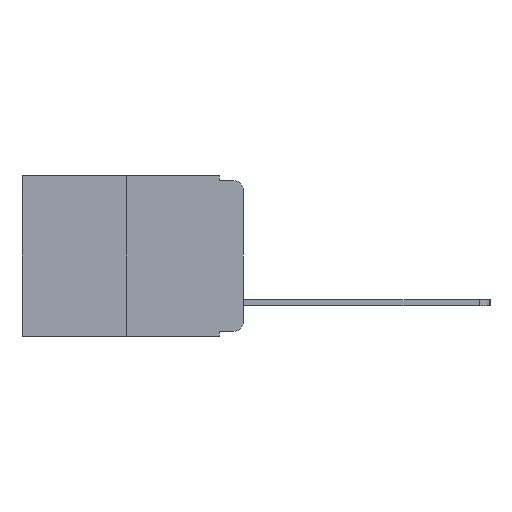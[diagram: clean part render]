
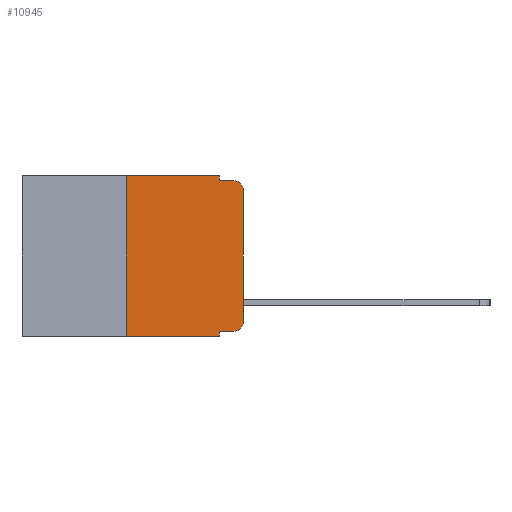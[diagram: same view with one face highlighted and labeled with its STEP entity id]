
A CAD part, left-side view. The second image highlights one B-rep face of the part: STEP entity #10945.
In plain terms, the highlighted planar face has unit normal (-1, 0, 0).
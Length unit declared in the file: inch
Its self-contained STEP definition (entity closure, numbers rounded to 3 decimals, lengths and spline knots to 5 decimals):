
#144 = EDGE_CURVE ( 'NONE', #13487, #6773, #2012, .T. ) ;
#500 = VERTEX_POINT ( 'NONE', #2441 ) ;
#527 = DIRECTION ( 'NONE',  ( 0., -1., 0. ) ) ;
#773 = AXIS2_PLACEMENT_3D ( 'NONE', #11230, #8162, #3846 ) ;
#955 = AXIS2_PLACEMENT_3D ( 'NONE', #4087, #8547, #12707 ) ;
#1427 = CARTESIAN_POINT ( 'NONE',  ( 0., 0.02, -0.01 ) ) ;
#2012 = LINE ( 'NONE', #13451, #7382 ) ;
#2046 = VERTEX_POINT ( 'NONE', #8762 ) ;
#2049 = DIRECTION ( 'NONE',  ( 0., -1., 0. ) ) ;
#2094 = LINE ( 'NONE', #11624, #9943 ) ;
#2283 = ORIENTED_EDGE ( 'NONE', *, *, #3135, .F. ) ;
#2360 = EDGE_LOOP ( 'NONE', ( #12227, #9770, #12539, #10143, #7335, #4859, #7635, #2283, #10321, #7983 ) ) ;
#2441 = CARTESIAN_POINT ( 'NONE',  ( 0., 0.25, -0.343 ) ) ;
#2463 = FACE_OUTER_BOUND ( 'NONE', #2360, .T. ) ;
#3135 = EDGE_CURVE ( 'NONE', #11764, #10428, #8601, .T. ) ;
#3271 = DIRECTION ( 'NONE',  ( 0., 0., 1. ) ) ;
#3550 = VECTOR ( 'NONE', #3271, 39.37008 ) ;
#3846 = DIRECTION ( 'NONE',  ( 0., 0., -1. ) ) ;
#3886 = EDGE_CURVE ( 'NONE', #10408, #6773, #5937, .T. ) ;
#4087 = CARTESIAN_POINT ( 'NONE',  ( 0., 0.473, 0. ) ) ;
#4218 = CARTESIAN_POINT ( 'NONE',  ( 0., 0.25, 0. ) ) ;
#4588 = CARTESIAN_POINT ( 'NONE',  ( 0., 0.02, -0.03 ) ) ;
#4742 = LINE ( 'NONE', #11142, #7216 ) ;
#4859 = ORIENTED_EDGE ( 'NONE', *, *, #9819, .F. ) ;
#4990 = DIRECTION ( 'NONE',  ( 0., 0., -1. ) ) ;
#5002 = DIRECTION ( 'NONE',  ( -1., 0., 0. ) ) ;
#5090 = DIRECTION ( 'NONE',  ( 0., -1., 0. ) ) ;
#5436 = DIRECTION ( 'NONE',  ( 0., 0., -1. ) ) ;
#5575 = VECTOR ( 'NONE', #12709, 39.37008 ) ;
#5848 = EDGE_CURVE ( 'NONE', #2046, #13487, #11241, .T. ) ;
#5937 = CIRCLE ( 'NONE', #10540, 0.02 ) ;
#6435 = EDGE_CURVE ( 'NONE', #500, #10428, #10713, .T. ) ;
#6773 = VERTEX_POINT ( 'NONE', #1427 ) ;
#7216 = VECTOR ( 'NONE', #11431, 39.37008 ) ;
#7335 = ORIENTED_EDGE ( 'NONE', *, *, #12509, .F. ) ;
#7382 = VECTOR ( 'NONE', #5090, 39.37008 ) ;
#7523 = PLANE ( 'NONE',  #955 ) ;
#7635 = ORIENTED_EDGE ( 'NONE', *, *, #6435, .T. ) ;
#7705 = CARTESIAN_POINT ( 'NONE',  ( 0., 0.051, -0.01 ) ) ;
#7826 = EDGE_CURVE ( 'NONE', #8843, #10408, #4742, .T. ) ;
#7895 = VECTOR ( 'NONE', #13499, 39.37008 ) ;
#7983 = ORIENTED_EDGE ( 'NONE', *, *, #10238, .T. ) ;
#7985 = VECTOR ( 'NONE', #5436, 39.37008 ) ;
#8162 = DIRECTION ( 'NONE',  ( -1., 0., 0. ) ) ;
#8256 = CARTESIAN_POINT ( 'NONE',  ( 0., 0.051, 0. ) ) ;
#8547 = DIRECTION ( 'NONE',  ( 1., 0., 0. ) ) ;
#8601 = LINE ( 'NONE', #12526, #7985 ) ;
#8762 = CARTESIAN_POINT ( 'NONE',  ( 0., 0.051, 0. ) ) ;
#8843 = VERTEX_POINT ( 'NONE', #9157 ) ;
#8940 = CIRCLE ( 'NONE', #773, 0.02 ) ;
#9144 = CARTESIAN_POINT ( 'NONE',  ( 0., 0.473, 0. ) ) ;
#9157 = CARTESIAN_POINT ( 'NONE',  ( 0., 0., -0.313 ) ) ;
#9770 = ORIENTED_EDGE ( 'NONE', *, *, #3886, .T. ) ;
#9819 = EDGE_CURVE ( 'NONE', #500, #9896, #11951, .T. ) ;
#9896 = VERTEX_POINT ( 'NONE', #4218 ) ;
#9943 = VECTOR ( 'NONE', #2049, 39.37008 ) ;
#9968 = VERTEX_POINT ( 'NONE', #10446 ) ;
#10143 = ORIENTED_EDGE ( 'NONE', *, *, #5848, .F. ) ;
#10238 = EDGE_CURVE ( 'NONE', #9968, #8843, #8940, .T. ) ;
#10321 = ORIENTED_EDGE ( 'NONE', *, *, #11403, .T. ) ;
#10408 = VERTEX_POINT ( 'NONE', #13414 ) ;
#10428 = VERTEX_POINT ( 'NONE', #11847 ) ;
#10446 = CARTESIAN_POINT ( 'NONE',  ( 0., 0.02, -0.333 ) ) ;
#10540 = AXIS2_PLACEMENT_3D ( 'NONE', #4588, #5002, #4990 ) ;
#10713 = LINE ( 'NONE', #12746, #7895 ) ;
#10741 = LINE ( 'NONE', #9144, #13122 ) ;
#10945 = ADVANCED_FACE ( 'NONE', ( #2463 ), #7523, .F. ) ;
#11142 = CARTESIAN_POINT ( 'NONE',  ( 0., 0., 0. ) ) ;
#11230 = CARTESIAN_POINT ( 'NONE',  ( 0., 0.02, -0.313 ) ) ;
#11241 = LINE ( 'NONE', #8256, #5575 ) ;
#11403 = EDGE_CURVE ( 'NONE', #11764, #9968, #2094, .T. ) ;
#11431 = DIRECTION ( 'NONE',  ( 0., 0., 1. ) ) ;
#11624 = CARTESIAN_POINT ( 'NONE',  ( 0., 0.051, -0.333 ) ) ;
#11764 = VERTEX_POINT ( 'NONE', #12279 ) ;
#11847 = CARTESIAN_POINT ( 'NONE',  ( 0., 0.051, -0.343 ) ) ;
#11951 = LINE ( 'NONE', #12108, #3550 ) ;
#12108 = CARTESIAN_POINT ( 'NONE',  ( 0., 0.25, 0. ) ) ;
#12227 = ORIENTED_EDGE ( 'NONE', *, *, #7826, .T. ) ;
#12279 = CARTESIAN_POINT ( 'NONE',  ( 0., 0.051, -0.333 ) ) ;
#12509 = EDGE_CURVE ( 'NONE', #9896, #2046, #10741, .T. ) ;
#12526 = CARTESIAN_POINT ( 'NONE',  ( 0., 0.051, 0. ) ) ;
#12539 = ORIENTED_EDGE ( 'NONE', *, *, #144, .F. ) ;
#12707 = DIRECTION ( 'NONE',  ( 0., 0., -1. ) ) ;
#12709 = DIRECTION ( 'NONE',  ( 0., 0., -1. ) ) ;
#12746 = CARTESIAN_POINT ( 'NONE',  ( 0., 0.473, -0.343 ) ) ;
#13122 = VECTOR ( 'NONE', #527, 39.37008 ) ;
#13414 = CARTESIAN_POINT ( 'NONE',  ( 0., 0., -0.03 ) ) ;
#13451 = CARTESIAN_POINT ( 'NONE',  ( 0., 0.051, -0.01 ) ) ;
#13487 = VERTEX_POINT ( 'NONE', #7705 ) ;
#13499 = DIRECTION ( 'NONE',  ( 0., -1., 0. ) ) ;
